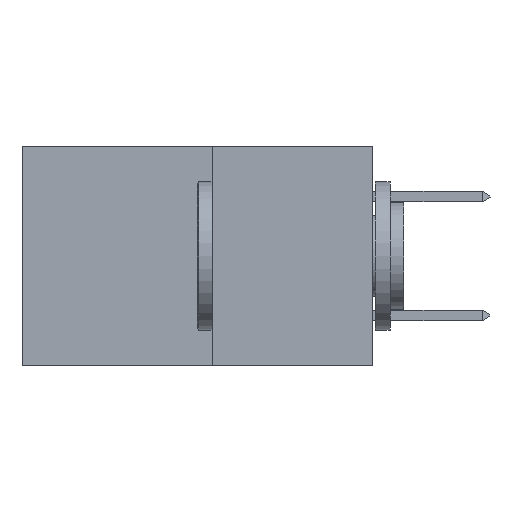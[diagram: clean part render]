
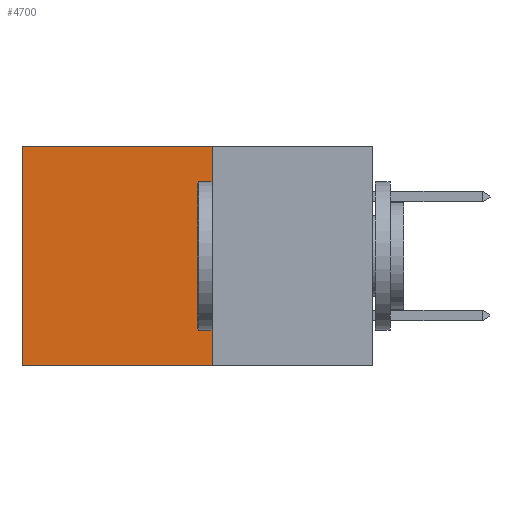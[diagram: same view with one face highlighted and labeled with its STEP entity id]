
A CAD part, left-side view. The second image highlights one B-rep face of the part: STEP entity #4700.
In plain terms, the highlighted planar face has unit normal (-1, 0, 0).
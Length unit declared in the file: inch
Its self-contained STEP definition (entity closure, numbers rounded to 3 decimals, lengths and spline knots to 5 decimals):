
#196 = CARTESIAN_POINT ( 'NONE',  ( 0.277, 0.59, 0. ) ) ;
#205 = EDGE_CURVE ( 'NONE', #4001, #5634, #9369, .T. ) ;
#486 = CARTESIAN_POINT ( 'NONE',  ( 0.277, 0.27, -0.37 ) ) ;
#645 = FACE_OUTER_BOUND ( 'NONE', #9585, .T. ) ;
#854 = CARTESIAN_POINT ( 'NONE',  ( 0.277, 0.27, -0.37 ) ) ;
#887 = DIRECTION ( 'NONE',  ( 1., 0., 0. ) ) ;
#911 = LINE ( 'NONE', #854, #2966 ) ;
#1270 = EDGE_CURVE ( 'NONE', #7355, #5634, #6771, .T. ) ;
#1655 = PLANE ( 'NONE',  #7163 ) ;
#1758 = VECTOR ( 'NONE', #6434, 39.37008 ) ;
#2101 = CARTESIAN_POINT ( 'NONE',  ( 0.277, 0.59, -0.37 ) ) ;
#2414 = ORIENTED_EDGE ( 'NONE', *, *, #2790, .T. ) ;
#2790 = EDGE_CURVE ( 'NONE', #5069, #7355, #4305, .T. ) ;
#2966 = VECTOR ( 'NONE', #6150, 39.37008 ) ;
#3041 = VECTOR ( 'NONE', #4102, 39.37008 ) ;
#3954 = ORIENTED_EDGE ( 'NONE', *, *, #4655, .F. ) ;
#4001 = VERTEX_POINT ( 'NONE', #486 ) ;
#4102 = DIRECTION ( 'NONE',  ( 0., 0., -1. ) ) ;
#4305 = LINE ( 'NONE', #9039, #7990 ) ;
#4655 = EDGE_CURVE ( 'NONE', #5069, #4001, #911, .T. ) ;
#4700 = ADVANCED_FACE ( 'NONE', ( #645 ), #1655, .F. ) ;
#5069 = VERTEX_POINT ( 'NONE', #8736 ) ;
#5634 = VERTEX_POINT ( 'NONE', #5732 ) ;
#5732 = CARTESIAN_POINT ( 'NONE',  ( 0.277, 0.59, -0.37 ) ) ;
#6150 = DIRECTION ( 'NONE',  ( 0., 0., -1. ) ) ;
#6187 = DIRECTION ( 'NONE',  ( 0., 0., -1. ) ) ;
#6434 = DIRECTION ( 'NONE',  ( 0., 1., 0. ) ) ;
#6732 = ORIENTED_EDGE ( 'NONE', *, *, #1270, .T. ) ;
#6771 = LINE ( 'NONE', #2101, #3041 ) ;
#7163 = AXIS2_PLACEMENT_3D ( 'NONE', #9046, #887, #6187 ) ;
#7296 = DIRECTION ( 'NONE',  ( 0., 1., 0. ) ) ;
#7355 = VERTEX_POINT ( 'NONE', #196 ) ;
#7990 = VECTOR ( 'NONE', #7296, 39.37008 ) ;
#8736 = CARTESIAN_POINT ( 'NONE',  ( 0.277, 0.27, 0. ) ) ;
#8872 = ORIENTED_EDGE ( 'NONE', *, *, #205, .F. ) ;
#8945 = CARTESIAN_POINT ( 'NONE',  ( 0.277, 0.27, -0.37 ) ) ;
#9039 = CARTESIAN_POINT ( 'NONE',  ( 0.277, 0.27, 0. ) ) ;
#9046 = CARTESIAN_POINT ( 'NONE',  ( 0.277, 0.27, -0.37 ) ) ;
#9369 = LINE ( 'NONE', #8945, #1758 ) ;
#9585 = EDGE_LOOP ( 'NONE', ( #6732, #8872, #3954, #2414 ) ) ;
